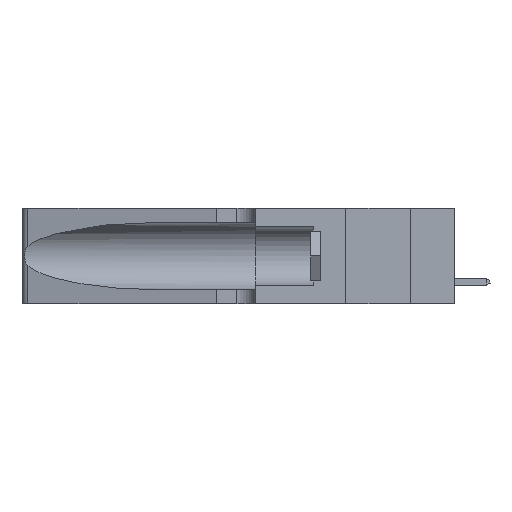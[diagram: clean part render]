
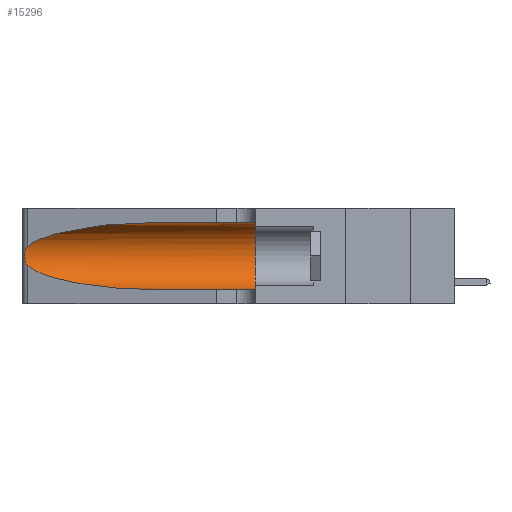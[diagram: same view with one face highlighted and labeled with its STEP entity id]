
A CAD part, left-side view. The second image highlights one B-rep face of the part: STEP entity #15296.
In plain terms, the highlighted cylindrical face has radius 3.308 mm (diameter 6.617 mm), a partial arc.
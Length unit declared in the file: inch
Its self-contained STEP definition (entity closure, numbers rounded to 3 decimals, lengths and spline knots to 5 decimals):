
#239 = CARTESIAN_POINT ( 'NONE',  ( 0.25787, 1.23484, 0.2124 ) ) ;
#444 = CARTESIAN_POINT ( 'NONE',  ( 0.1305, 1.61858, 0.185 ) ) ;
#620 = ORIENTED_EDGE ( 'NONE', *, *, #2110, .T. ) ;
#706 = CARTESIAN_POINT ( 'NONE',  ( 0.1305, 0.72297, 0.31525 ) ) ;
#710 = CARTESIAN_POINT ( 'NONE',  ( 0.25789, 1.23486, 0.15765 ) ) ;
#1412 = EDGE_CURVE ( 'NONE', #15234, #12554, #9785, .T. ) ;
#1416 = DIRECTION ( 'NONE',  ( 0., -1., 0. ) ) ;
#2001 = DIRECTION ( 'NONE',  ( 0., -1., 0. ) ) ;
#2110 = EDGE_CURVE ( 'NONE', #12554, #15267, #11840, .T. ) ;
#2176 = CARTESIAN_POINT ( 'NONE',  ( 0.25487, 1.22718, 0.22369 ) ) ;
#2201 = ORIENTED_EDGE ( 'NONE', *, *, #13183, .T. ) ;
#2384 = CARTESIAN_POINT ( 'NONE',  ( 0.25555, 1.22993, 0.14849 ) ) ;
#2463 =( BOUNDED_CURVE ( )  B_SPLINE_CURVE ( 3, ( #706, #8186, #3652, #4964 ),
 .UNSPECIFIED., .F., .F. ) 
 B_SPLINE_CURVE_WITH_KNOTS ( ( 4, 4 ),
 ( 1.5708, 2.84003 ),
 .UNSPECIFIED. ) 
 CURVE ( )  GEOMETRIC_REPRESENTATION_ITEM ( )  RATIONAL_B_SPLINE_CURVE ( ( 1., 0.87, 0.87, 1. ) ) 
 REPRESENTATION_ITEM ( '' )  );
#2963 = CARTESIAN_POINT ( 'NONE',  ( 0.1305, 0.72297, 0.05475 ) ) ;
#3386 = CARTESIAN_POINT ( 'NONE',  ( 0.25854, 1.2359, 0.20912 ) ) ;
#3522 = DIRECTION ( 'NONE',  ( 0., -1., 0. ) ) ;
#3652 = CARTESIAN_POINT ( 'NONE',  ( 0.2373, 1.15595, 0.28018 ) ) ;
#3669 = CYLINDRICAL_SURFACE ( 'NONE', #15298, 0.13025 ) ;
#3804 = AXIS2_PLACEMENT_3D ( 'NONE', #12866, #6664, #6743 ) ;
#3972 = VERTEX_POINT ( 'NONE', #16795 ) ;
#4964 = CARTESIAN_POINT ( 'NONE',  ( 0.25487, 1.22718, 0.22369 ) ) ;
#5284 = CARTESIAN_POINT ( 'NONE',  ( 0.25639, 1.23186, 0.15144 ) ) ;
#5981 = CARTESIAN_POINT ( 'NONE',  ( 0.1305, 0.35, 0.31525 ) ) ;
#6493 = CARTESIAN_POINT ( 'NONE',  ( 0.25639, 1.23184, 0.21858 ) ) ;
#6664 = DIRECTION ( 'NONE',  ( 0., 1., 0. ) ) ;
#6743 = DIRECTION ( 'NONE',  ( 0., 0., 1. ) ) ;
#6840 = EDGE_CURVE ( 'NONE', #17597, #13719, #15445, .T. ) ;
#7974 = FACE_OUTER_BOUND ( 'NONE', #10111, .T. ) ;
#7993 = CARTESIAN_POINT ( 'NONE',  ( 0.26018, 1.23835, 0.19895 ) ) ;
#8137 = CARTESIAN_POINT ( 'NONE',  ( 0.1305, 1.61858, 0.31525 ) ) ;
#8186 = CARTESIAN_POINT ( 'NONE',  ( 0.18966, 0.96281, 0.31525 ) ) ;
#8248 = CARTESIAN_POINT ( 'NONE',  ( 0.1305, 0.72297, 0.05475 ) ) ;
#9509 = CARTESIAN_POINT ( 'NONE',  ( 0.26075, 1.23896, 0.178 ) ) ;
#9521 = CARTESIAN_POINT ( 'NONE',  ( 0.25487, 1.22718, 0.14631 ) ) ;
#9785 = B_SPLINE_CURVE_WITH_KNOTS ( 'NONE', 3,
 ( #12676, #16933, #6493, #239, #3386, #7993, #18618, #9509, #11035, #9844, #710, #5284, #2384, #11360 ),
 .UNSPECIFIED., .F., .F.,
 ( 4, 2, 2, 2, 2, 2, 4 ),
 ( 0., 0.00027, 0.00053, 0.00107, 0.0016, 0.00187, 0.00214 ),
 .UNSPECIFIED. ) ;
#9844 = CARTESIAN_POINT ( 'NONE',  ( 0.25856, 1.23593, 0.16098 ) ) ;
#10111 = EDGE_LOOP ( 'NONE', ( #2201, #19312, #620, #14403, #16908, #19300 ) ) ;
#10610 = CARTESIAN_POINT ( 'NONE',  ( 0.1305, 1.61858, 0.05475 ) ) ;
#11035 = CARTESIAN_POINT ( 'NONE',  ( 0.26017, 1.23833, 0.17102 ) ) ;
#11337 = EDGE_CURVE ( 'NONE', #13719, #3972, #13539, .T. ) ;
#11360 = CARTESIAN_POINT ( 'NONE',  ( 0.25487, 1.22718, 0.14631 ) ) ;
#11681 = LINE ( 'NONE', #10610, #18081 ) ;
#11840 =( BOUNDED_CURVE ( )  B_SPLINE_CURVE ( 3, ( #11929, #16439, #16712, #2963 ),
 .UNSPECIFIED., .F., .F. ) 
 B_SPLINE_CURVE_WITH_KNOTS ( ( 4, 4 ),
 ( 3.44316, 4.71239 ),
 .UNSPECIFIED. ) 
 CURVE ( )  GEOMETRIC_REPRESENTATION_ITEM ( )  RATIONAL_B_SPLINE_CURVE ( ( 1., 0.87, 0.87, 1. ) ) 
 REPRESENTATION_ITEM ( '' )  );
#11929 = CARTESIAN_POINT ( 'NONE',  ( 0.25487, 1.22718, 0.14631 ) ) ;
#12554 = VERTEX_POINT ( 'NONE', #9521 ) ;
#12676 = CARTESIAN_POINT ( 'NONE',  ( 0.25487, 1.22718, 0.22369 ) ) ;
#12866 = CARTESIAN_POINT ( 'NONE',  ( 0.1305, 0.35, 0.185 ) ) ;
#13183 = EDGE_CURVE ( 'NONE', #17597, #15234, #2463, .T. ) ;
#13277 = VECTOR ( 'NONE', #2001, 39.37008 ) ;
#13539 = CIRCLE ( 'NONE', #3804, 0.13025 ) ;
#13719 = VERTEX_POINT ( 'NONE', #5981 ) ;
#14135 = DIRECTION ( 'NONE',  ( 0., 0., -1. ) ) ;
#14403 = ORIENTED_EDGE ( 'NONE', *, *, #16855, .T. ) ;
#15234 = VERTEX_POINT ( 'NONE', #2176 ) ;
#15267 = VERTEX_POINT ( 'NONE', #8248 ) ;
#15296 = ADVANCED_FACE ( 'NONE', ( #7974 ), #3669, .F. ) ;
#15298 = AXIS2_PLACEMENT_3D ( 'NONE', #444, #3522, #14135 ) ;
#15445 = LINE ( 'NONE', #8137, #13277 ) ;
#16439 = CARTESIAN_POINT ( 'NONE',  ( 0.2373, 1.15595, 0.08982 ) ) ;
#16712 = CARTESIAN_POINT ( 'NONE',  ( 0.18966, 0.96281, 0.05475 ) ) ;
#16795 = CARTESIAN_POINT ( 'NONE',  ( 0.1305, 0.35, 0.05475 ) ) ;
#16855 = EDGE_CURVE ( 'NONE', #15267, #3972, #11681, .T. ) ;
#16908 = ORIENTED_EDGE ( 'NONE', *, *, #11337, .F. ) ;
#16933 = CARTESIAN_POINT ( 'NONE',  ( 0.25555, 1.22994, 0.2215 ) ) ;
#17597 = VERTEX_POINT ( 'NONE', #18706 ) ;
#18081 = VECTOR ( 'NONE', #1416, 39.37008 ) ;
#18618 = CARTESIAN_POINT ( 'NONE',  ( 0.26075, 1.23896, 0.19203 ) ) ;
#18706 = CARTESIAN_POINT ( 'NONE',  ( 0.1305, 0.72297, 0.31525 ) ) ;
#19300 = ORIENTED_EDGE ( 'NONE', *, *, #6840, .F. ) ;
#19312 = ORIENTED_EDGE ( 'NONE', *, *, #1412, .T. ) ;
